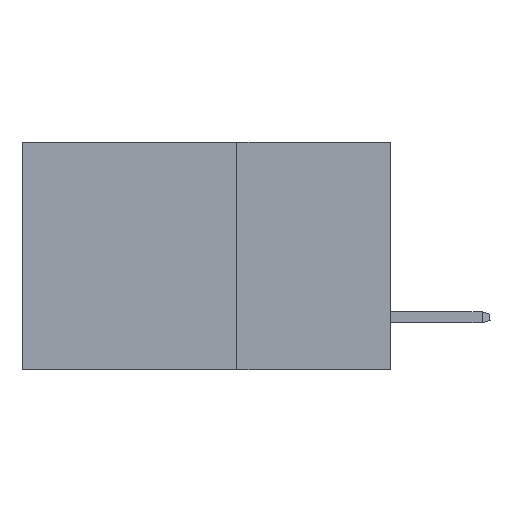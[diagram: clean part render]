
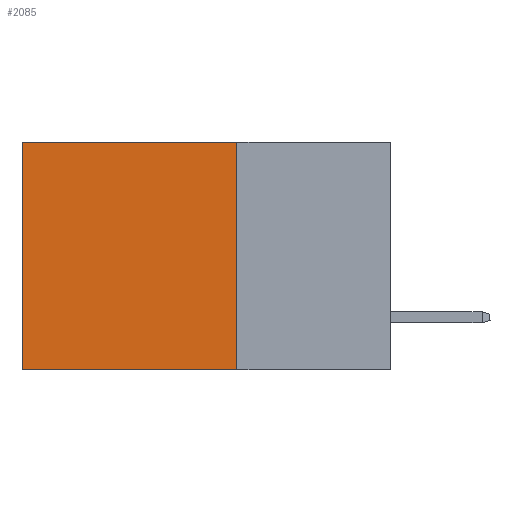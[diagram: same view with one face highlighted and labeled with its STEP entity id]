
A CAD part, left-side view. The second image highlights one B-rep face of the part: STEP entity #2085.
In plain terms, the highlighted planar face has unit normal (-1, 0, 0).
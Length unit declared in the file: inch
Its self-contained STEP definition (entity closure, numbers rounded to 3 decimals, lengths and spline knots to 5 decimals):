
#1786 = CARTESIAN_POINT ( 'NONE',  ( 0.2875, 0.6, 0. ) ) ;
#1902 = CARTESIAN_POINT ( 'NONE',  ( 0.2875, 0.25, 0. ) ) ;
#2085 = ADVANCED_FACE ( 'NONE', ( #16947 ), #5856, .F. ) ;
#2679 = VECTOR ( 'NONE', #20735, 39.37008 ) ;
#3895 = VERTEX_POINT ( 'NONE', #14185 ) ;
#3933 = CARTESIAN_POINT ( 'NONE',  ( 0.2875, 0.25, 0. ) ) ;
#3959 = EDGE_CURVE ( 'NONE', #21536, #20156, #20773, .T. ) ;
#5648 = EDGE_CURVE ( 'NONE', #3895, #21013, #14737, .T. ) ;
#5856 = PLANE ( 'NONE',  #7736 ) ;
#6019 = DIRECTION ( 'NONE',  ( 0., 0., -1. ) ) ;
#6990 = VECTOR ( 'NONE', #18991, 39.37008 ) ;
#7736 = AXIS2_PLACEMENT_3D ( 'NONE', #15704, #12847, #6019 ) ;
#9223 = ORIENTED_EDGE ( 'NONE', *, *, #14039, .F. ) ;
#9655 = CARTESIAN_POINT ( 'NONE',  ( 0.2875, 0.6, -0.37 ) ) ;
#11269 = DIRECTION ( 'NONE',  ( 0., 1., 0. ) ) ;
#11765 = EDGE_LOOP ( 'NONE', ( #17079, #12304, #9223, #17344 ) ) ;
#12264 = VECTOR ( 'NONE', #15885, 39.37008 ) ;
#12304 = ORIENTED_EDGE ( 'NONE', *, *, #3959, .F. ) ;
#12847 = DIRECTION ( 'NONE',  ( 1., 0., 0. ) ) ;
#13772 = CARTESIAN_POINT ( 'NONE',  ( 0.2875, 0.25, -0.37 ) ) ;
#14039 = EDGE_CURVE ( 'NONE', #3895, #21536, #16876, .T. ) ;
#14185 = CARTESIAN_POINT ( 'NONE',  ( 0.2875, 0.25, 0. ) ) ;
#14737 = LINE ( 'NONE', #3933, #16111 ) ;
#15704 = CARTESIAN_POINT ( 'NONE',  ( 0.2875, 0.25, 0. ) ) ;
#15885 = DIRECTION ( 'NONE',  ( 0., 0., -1. ) ) ;
#16111 = VECTOR ( 'NONE', #11269, 39.37008 ) ;
#16295 = CARTESIAN_POINT ( 'NONE',  ( 0.2875, 0.25, -0.37 ) ) ;
#16393 = EDGE_CURVE ( 'NONE', #21013, #20156, #19175, .T. ) ;
#16876 = LINE ( 'NONE', #1902, #12264 ) ;
#16947 = FACE_OUTER_BOUND ( 'NONE', #11765, .T. ) ;
#17079 = ORIENTED_EDGE ( 'NONE', *, *, #16393, .T. ) ;
#17344 = ORIENTED_EDGE ( 'NONE', *, *, #5648, .T. ) ;
#18991 = DIRECTION ( 'NONE',  ( 0., 1., 0. ) ) ;
#19175 = LINE ( 'NONE', #1786, #2679 ) ;
#20140 = CARTESIAN_POINT ( 'NONE',  ( 0.2875, 0.6, 0. ) ) ;
#20156 = VERTEX_POINT ( 'NONE', #9655 ) ;
#20735 = DIRECTION ( 'NONE',  ( 0., 0., -1. ) ) ;
#20773 = LINE ( 'NONE', #13772, #6990 ) ;
#21013 = VERTEX_POINT ( 'NONE', #20140 ) ;
#21536 = VERTEX_POINT ( 'NONE', #16295 ) ;
